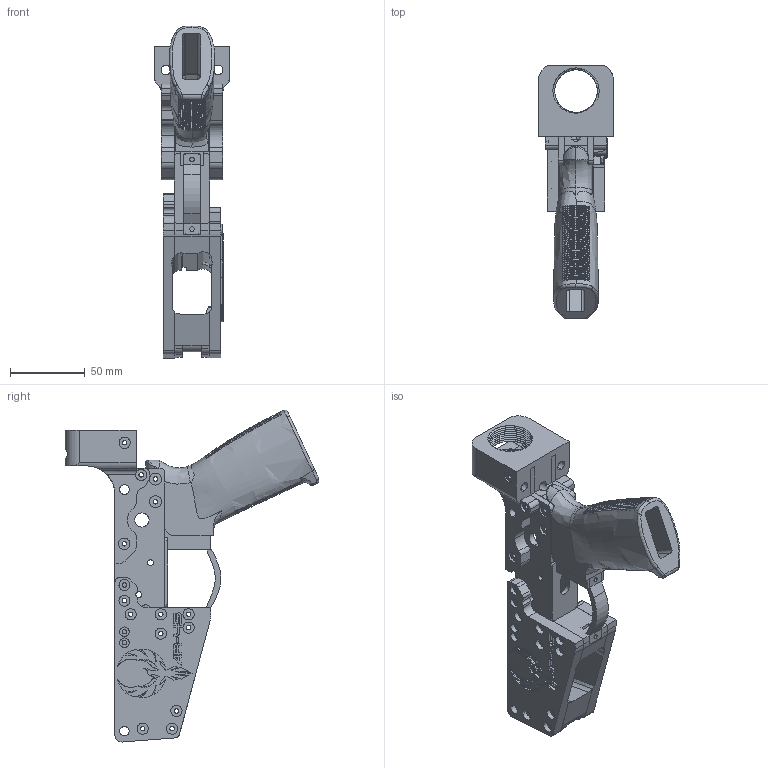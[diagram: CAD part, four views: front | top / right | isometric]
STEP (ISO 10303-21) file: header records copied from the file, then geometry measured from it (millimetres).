
FILE_DESCRIPTION (( 'STEP AP214' ), '1' );
FILE_NAME ('Firebolt_45_UBolt.STEP', '2020-12-05T18:49:06', ( '' ), ( '' ), 'SwSTEP 2.0', 'SolidWorks 2020', '' );
FILE_SCHEMA (( 'AUTOMOTIVE_DESIGN' ));
Length unit declared in the file: millimetre
Products named in the file (13): Firebolt_45_Mag_Well_Rear; Firebolt_UBolt_Buffer_Tower; Mag_Release; Firebolt_Fire_Control_Well_Bottom; Firebolt_45_Mag_Well_Front; Firebolt_UBolt_Side_Left; Firebolt_UBolt_Side_Right; Firebolt_45_Mag_Well_Right; Firebolt_UBolt_Grip_Part; Firebolt_Trigger_Guard; Firebolt_UBolt_Pistol_Grip; Firebolt_45_UBolt; Firebolt_45_Mag_Well_Left
Assembly tree (12 placements, depth 2):
  Firebolt_45_UBolt
    Firebolt_UBolt_Buffer_Tower
    Firebolt_UBolt_Side_Left
    Firebolt_UBolt_Side_Right
    Firebolt_UBolt_Grip_Part
    Firebolt_UBolt_Pistol_Grip
    Firebolt_Fire_Control_Well_Bottom
    Firebolt_Trigger_Guard
    Firebolt_45_Mag_Well_Rear
    Firebolt_45_Mag_Well_Right
    Firebolt_45_Mag_Well_Left
    Firebolt_45_Mag_Well_Front
    Mag_Release
Bounding box: 50 x 170.14 x 222.58 mm (x, y, z)
Volume: 293533.8 mm3; surface area: 127576.8 mm2
Topology: 12 solids, 12 shells, 2377 faces, 7146 edges, 4831 vertices
Faces by surface type: plane 1565, cylinder 486, bspline 294, cone 19, sphere 7, torus 6
Entity records: 147075 total; most frequent: CARTESIAN_POINT 85631, ORIENTED_EDGE 14282, DIRECTION 10341, EDGE_CURVE 7141, VERTEX_POINT 4831, LINE 4421, VECTOR 4421, AXIS2_PLACEMENT_3D 2960
